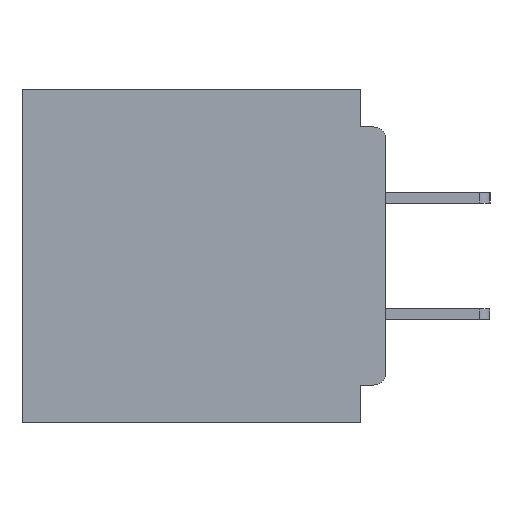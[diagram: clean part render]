
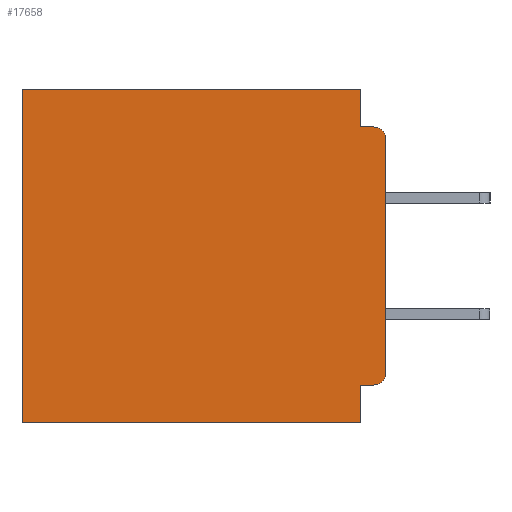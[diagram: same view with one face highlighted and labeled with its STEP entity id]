
A CAD part, left-side view. The second image highlights one B-rep face of the part: STEP entity #17658.
In plain terms, the highlighted planar face has unit normal (-1, 0, 0).
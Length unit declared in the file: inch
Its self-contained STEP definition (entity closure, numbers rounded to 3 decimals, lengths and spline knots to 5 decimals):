
#1189 = LINE ( 'NONE', #3305, #39046 ) ;
#1204 = DIRECTION ( 'NONE',  ( 0., 0., -1. ) ) ;
#1219 = VERTEX_POINT ( 'NONE', #9937 ) ;
#1847 = EDGE_CURVE ( 'NONE', #13124, #15725, #2911, .T. ) ;
#2742 = ORIENTED_EDGE ( 'NONE', *, *, #39844, .T. ) ;
#2902 = CARTESIAN_POINT ( 'NONE',  ( 0.3, 0.031, -0.4 ) ) ;
#2911 = LINE ( 'NONE', #22885, #54415 ) ;
#3104 = LINE ( 'NONE', #55342, #40917 ) ;
#3171 = DIRECTION ( 'NONE',  ( 0., 1., 0. ) ) ;
#3269 = DIRECTION ( 'NONE',  ( -1., 0., 0. ) ) ;
#3305 = CARTESIAN_POINT ( 'NONE',  ( 0.3, 0., -0.045 ) ) ;
#5848 = CIRCLE ( 'NONE', #60774, 0.015 ) ;
#6248 = VERTEX_POINT ( 'NONE', #55394 ) ;
#6568 = EDGE_CURVE ( 'NONE', #1219, #15725, #49010, .T. ) ;
#6896 = AXIS2_PLACEMENT_3D ( 'NONE', #34441, #8986, #45063 ) ;
#7472 = DIRECTION ( 'NONE',  ( 0., 1., 0. ) ) ;
#7777 = CIRCLE ( 'NONE', #53228, 0.015 ) ;
#8068 = EDGE_CURVE ( 'NONE', #28011, #1219, #9739, .T. ) ;
#8448 = DIRECTION ( 'NONE',  ( 0., -1., 0. ) ) ;
#8986 = DIRECTION ( 'NONE',  ( 1., 0., 0. ) ) ;
#9739 = LINE ( 'NONE', #33746, #62922 ) ;
#9937 = CARTESIAN_POINT ( 'NONE',  ( 0.3, 0.437, 0. ) ) ;
#10737 = ORIENTED_EDGE ( 'NONE', *, *, #13838, .F. ) ;
#11630 = CARTESIAN_POINT ( 'NONE',  ( 0.3, 0.437, -0.4 ) ) ;
#12374 = CARTESIAN_POINT ( 'NONE',  ( 0.3, 0.015, -0.045 ) ) ;
#12596 = VECTOR ( 'NONE', #56169, 39.37008 ) ;
#13124 = VERTEX_POINT ( 'NONE', #33727 ) ;
#13838 = EDGE_CURVE ( 'NONE', #35070, #52650, #1189, .T. ) ;
#14553 = EDGE_LOOP ( 'NONE', ( #33383, #49386, #10737, #56529, #40328, #46014, #29714, #54547, #23764, #2742 ) ) ;
#14926 = CARTESIAN_POINT ( 'NONE',  ( 0.3, 0., -0.4 ) ) ;
#15725 = VERTEX_POINT ( 'NONE', #21405 ) ;
#15752 = EDGE_CURVE ( 'NONE', #22411, #52650, #5848, .T. ) ;
#17658 = ADVANCED_FACE ( 'NONE', ( #62769 ), #49963, .F. ) ;
#18206 = EDGE_CURVE ( 'NONE', #28011, #35070, #3104, .T. ) ;
#21405 = CARTESIAN_POINT ( 'NONE',  ( 0.3, 0.437, -0.4 ) ) ;
#21727 = DIRECTION ( 'NONE',  ( 0., 0., -1. ) ) ;
#22411 = VERTEX_POINT ( 'NONE', #47890 ) ;
#22574 = VECTOR ( 'NONE', #23531, 39.37008 ) ;
#22885 = CARTESIAN_POINT ( 'NONE',  ( 0.3, 0., -0.4 ) ) ;
#23531 = DIRECTION ( 'NONE',  ( 0., 0., -1. ) ) ;
#23764 = ORIENTED_EDGE ( 'NONE', *, *, #51681, .F. ) ;
#24231 = LINE ( 'NONE', #2902, #22574 ) ;
#27835 = CARTESIAN_POINT ( 'NONE',  ( 0.3, 0., -0.355 ) ) ;
#28011 = VERTEX_POINT ( 'NONE', #34911 ) ;
#29714 = ORIENTED_EDGE ( 'NONE', *, *, #1847, .F. ) ;
#30722 = CARTESIAN_POINT ( 'NONE',  ( 0.3, 0.031, -0.045 ) ) ;
#31965 = DIRECTION ( 'NONE',  ( -1., 0., 0. ) ) ;
#32247 = VECTOR ( 'NONE', #48316, 39.37008 ) ;
#33383 = ORIENTED_EDGE ( 'NONE', *, *, #54146, .F. ) ;
#33727 = CARTESIAN_POINT ( 'NONE',  ( 0.3, 0.031, -0.4 ) ) ;
#33746 = CARTESIAN_POINT ( 'NONE',  ( 0.3, 0., 0. ) ) ;
#34070 = CARTESIAN_POINT ( 'NONE',  ( 0.3, 0.015, -0.34 ) ) ;
#34441 = CARTESIAN_POINT ( 'NONE',  ( 0.3, 0., -0.4 ) ) ;
#34621 = DIRECTION ( 'NONE',  ( 0., 0., -1. ) ) ;
#34911 = CARTESIAN_POINT ( 'NONE',  ( 0.3, 0.031, 0. ) ) ;
#35070 = VERTEX_POINT ( 'NONE', #30722 ) ;
#39046 = VECTOR ( 'NONE', #8448, 39.37008 ) ;
#39275 = DIRECTION ( 'NONE',  ( 0., 0., -1. ) ) ;
#39844 = EDGE_CURVE ( 'NONE', #44830, #6248, #7777, .T. ) ;
#40328 = ORIENTED_EDGE ( 'NONE', *, *, #8068, .T. ) ;
#40917 = VECTOR ( 'NONE', #34621, 39.37008 ) ;
#41973 = CARTESIAN_POINT ( 'NONE',  ( 0.3, 0.031, -0.355 ) ) ;
#44830 = VERTEX_POINT ( 'NONE', #66424 ) ;
#45063 = DIRECTION ( 'NONE',  ( 0., 0., -1. ) ) ;
#46014 = ORIENTED_EDGE ( 'NONE', *, *, #6568, .T. ) ;
#47890 = CARTESIAN_POINT ( 'NONE',  ( 0.3, 0., -0.06 ) ) ;
#48316 = DIRECTION ( 'NONE',  ( 0., 1., 0. ) ) ;
#49010 = LINE ( 'NONE', #11630, #55491 ) ;
#49386 = ORIENTED_EDGE ( 'NONE', *, *, #15752, .T. ) ;
#49963 = PLANE ( 'NONE',  #6896 ) ;
#51681 = EDGE_CURVE ( 'NONE', #44830, #63287, #58107, .T. ) ;
#52650 = VERTEX_POINT ( 'NONE', #12374 ) ;
#53228 = AXIS2_PLACEMENT_3D ( 'NONE', #34070, #3269, #39275 ) ;
#53698 = LINE ( 'NONE', #14926, #12596 ) ;
#54146 = EDGE_CURVE ( 'NONE', #22411, #6248, #53698, .T. ) ;
#54415 = VECTOR ( 'NONE', #7472, 39.37008 ) ;
#54547 = ORIENTED_EDGE ( 'NONE', *, *, #66268, .F. ) ;
#55342 = CARTESIAN_POINT ( 'NONE',  ( 0.3, 0.031, 0. ) ) ;
#55394 = CARTESIAN_POINT ( 'NONE',  ( 0.3, 0., -0.34 ) ) ;
#55491 = VECTOR ( 'NONE', #21727, 39.37008 ) ;
#56169 = DIRECTION ( 'NONE',  ( 0., 0., -1. ) ) ;
#56529 = ORIENTED_EDGE ( 'NONE', *, *, #18206, .F. ) ;
#58107 = LINE ( 'NONE', #27835, #32247 ) ;
#60774 = AXIS2_PLACEMENT_3D ( 'NONE', #62877, #31965, #1204 ) ;
#62769 = FACE_OUTER_BOUND ( 'NONE', #14553, .T. ) ;
#62877 = CARTESIAN_POINT ( 'NONE',  ( 0.3, 0.015, -0.06 ) ) ;
#62922 = VECTOR ( 'NONE', #3171, 39.37008 ) ;
#63287 = VERTEX_POINT ( 'NONE', #41973 ) ;
#66268 = EDGE_CURVE ( 'NONE', #63287, #13124, #24231, .T. ) ;
#66424 = CARTESIAN_POINT ( 'NONE',  ( 0.3, 0.015, -0.355 ) ) ;
